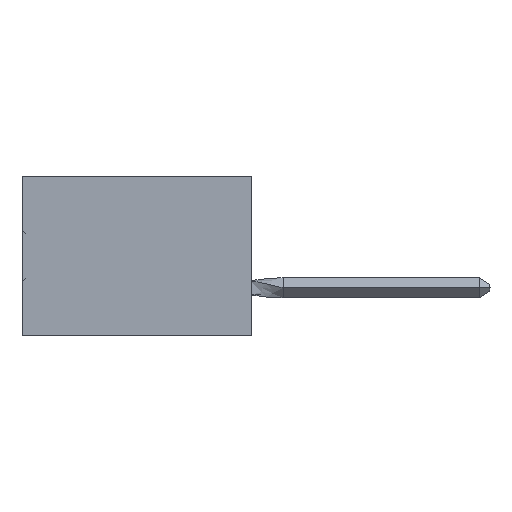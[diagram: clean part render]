
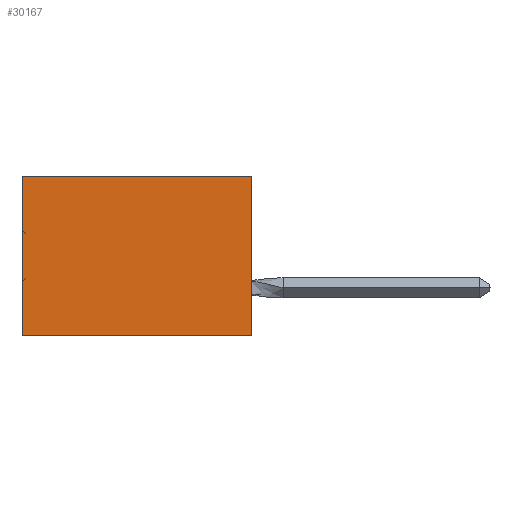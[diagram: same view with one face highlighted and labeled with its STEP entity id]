
A CAD part, left-side view. The second image highlights one B-rep face of the part: STEP entity #30167.
In plain terms, the highlighted planar face has unit normal (-1, 0, 0).
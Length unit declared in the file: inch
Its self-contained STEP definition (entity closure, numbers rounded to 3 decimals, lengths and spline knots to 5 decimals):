
#418 = CARTESIAN_POINT ( 'NONE',  ( 0.305, 0.72, -0.5 ) ) ;
#1148 = ORIENTED_EDGE ( 'NONE', *, *, #56067, .T. ) ;
#3618 = VECTOR ( 'NONE', #55395, 39.37008 ) ;
#10772 = CARTESIAN_POINT ( 'NONE',  ( 0.305, 0., -0.5 ) ) ;
#11962 = VERTEX_POINT ( 'NONE', #27309 ) ;
#12210 = CARTESIAN_POINT ( 'NONE',  ( 0.305, 0., 0. ) ) ;
#12784 = VECTOR ( 'NONE', #53065, 39.37008 ) ;
#19973 = DIRECTION ( 'NONE',  ( 0., 0., -1. ) ) ;
#21412 = EDGE_CURVE ( 'NONE', #27054, #44582, #34322, .T. ) ;
#22474 = CARTESIAN_POINT ( 'NONE',  ( 0.305, 0., -0.5 ) ) ;
#25324 = EDGE_CURVE ( 'NONE', #11962, #25563, #30941, .T. ) ;
#25563 = VERTEX_POINT ( 'NONE', #57372 ) ;
#25947 = VECTOR ( 'NONE', #50282, 39.37008 ) ;
#26496 = ORIENTED_EDGE ( 'NONE', *, *, #25324, .T. ) ;
#27054 = VERTEX_POINT ( 'NONE', #12210 ) ;
#27309 = CARTESIAN_POINT ( 'NONE',  ( 0.305, 0.72, 0. ) ) ;
#30167 = ADVANCED_FACE ( 'NONE', ( #40765 ), #33512, .F. ) ;
#30941 = LINE ( 'NONE', #418, #25947 ) ;
#31455 = EDGE_CURVE ( 'NONE', #44582, #25563, #42057, .T. ) ;
#33131 = ORIENTED_EDGE ( 'NONE', *, *, #31455, .F. ) ;
#33512 = PLANE ( 'NONE',  #44414 ) ;
#33518 = VECTOR ( 'NONE', #52533, 39.37008 ) ;
#34322 = LINE ( 'NONE', #46841, #3618 ) ;
#37119 = LINE ( 'NONE', #57674, #12784 ) ;
#40765 = FACE_OUTER_BOUND ( 'NONE', #43156, .T. ) ;
#42057 = LINE ( 'NONE', #52933, #33518 ) ;
#43156 = EDGE_LOOP ( 'NONE', ( #26496, #33131, #45743, #1148 ) ) ;
#44414 = AXIS2_PLACEMENT_3D ( 'NONE', #10772, #52409, #19973 ) ;
#44582 = VERTEX_POINT ( 'NONE', #22474 ) ;
#45743 = ORIENTED_EDGE ( 'NONE', *, *, #21412, .F. ) ;
#46841 = CARTESIAN_POINT ( 'NONE',  ( 0.305, 0., -0.5 ) ) ;
#50282 = DIRECTION ( 'NONE',  ( 0., 0., -1. ) ) ;
#52409 = DIRECTION ( 'NONE',  ( 1., 0., 0. ) ) ;
#52533 = DIRECTION ( 'NONE',  ( 0., 1., 0. ) ) ;
#52933 = CARTESIAN_POINT ( 'NONE',  ( 0.305, 0., -0.5 ) ) ;
#53065 = DIRECTION ( 'NONE',  ( 0., 1., 0. ) ) ;
#55395 = DIRECTION ( 'NONE',  ( 0., 0., -1. ) ) ;
#56067 = EDGE_CURVE ( 'NONE', #27054, #11962, #37119, .T. ) ;
#57372 = CARTESIAN_POINT ( 'NONE',  ( 0.305, 0.72, -0.5 ) ) ;
#57674 = CARTESIAN_POINT ( 'NONE',  ( 0.305, 0., 0. ) ) ;
